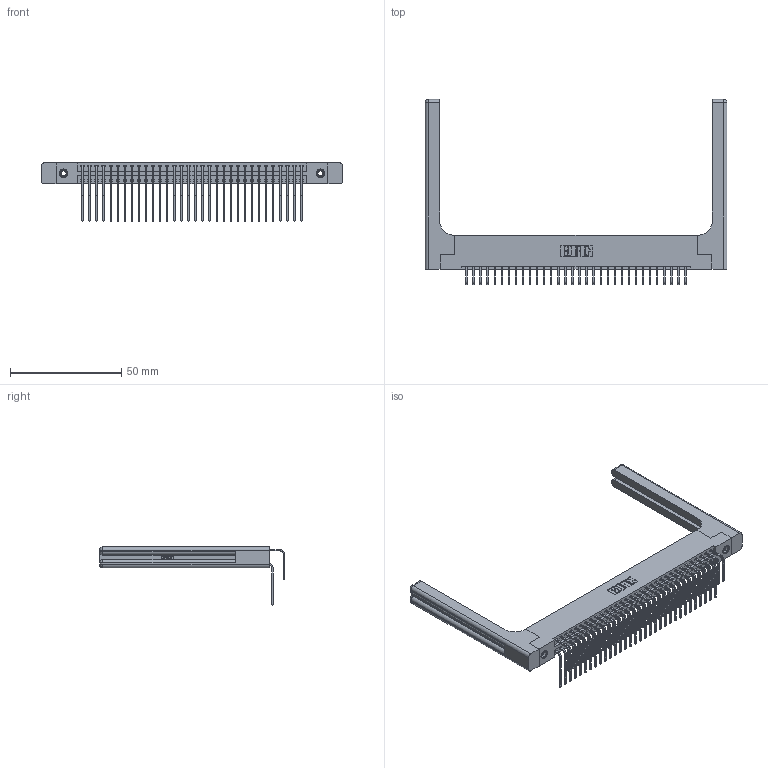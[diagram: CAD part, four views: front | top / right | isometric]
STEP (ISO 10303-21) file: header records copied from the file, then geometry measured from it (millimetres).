
FILE_DESCRIPTION (( 'STEP AP203' ), '1' );
FILE_NAME ('396-064-558-258.STEP', '2019-11-03T10:16:53', ( '' ), ( '' ), 'SwSTEP 2.0', 'SolidWorks 2016', '' );
FILE_SCHEMA (( 'CONFIG_CONTROL_DESIGN' ));
Length unit declared in the file: inch
Products named in the file (6): 346 Part_Flush Mounting Lugs - 0.156 Dia-TH; 345-292-001_558 Tail - 2; 396-064-558-258; 345-250-001_345-250-001-102; 345-292-001_558 559 Tail - 1; 346-220-058_345-220-058
Assembly tree (69 placements, depth 2):
  396-064-558-258
    346 Part_Flush Mounting Lugs - 0.156 Dia-TH
    345-292-001_558 559 Tail - 1  x32
    345-292-001_558 Tail - 2  x32
    345-250-001_345-250-001-102  x2
    346-220-058_345-220-058  x2
Bounding box: 135.66 x 83.12 x 26.16 mm (x, y, z)
Volume: 21014.4 mm3; surface area: 25171.2 mm2
Topology: 69 solids, 69 shells, 3834 faces, 11299 edges, 7426 vertices
Faces by surface type: plane 2592, cylinder 1182, bspline 36, cone 12, sphere 8, torus 4
Entity records: 29196 total; most frequent: CARTESIAN_POINT 5884, ORIENTED_EDGE 4564, DIRECTION 4142, EDGE_CURVE 2282, LINE 1890, VECTOR 1890, VERTEX_POINT 1510, AXIS2_PLACEMENT_3D 1126
